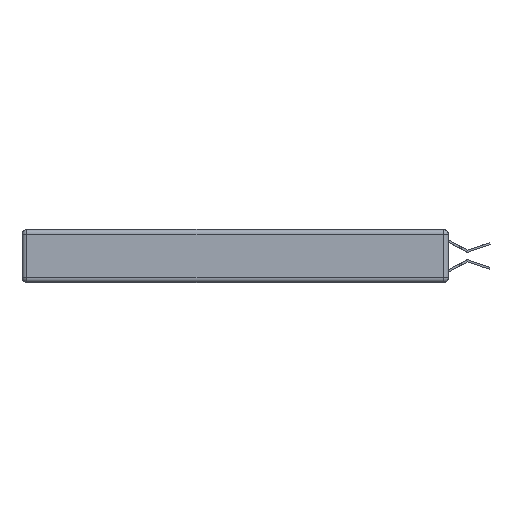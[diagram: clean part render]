
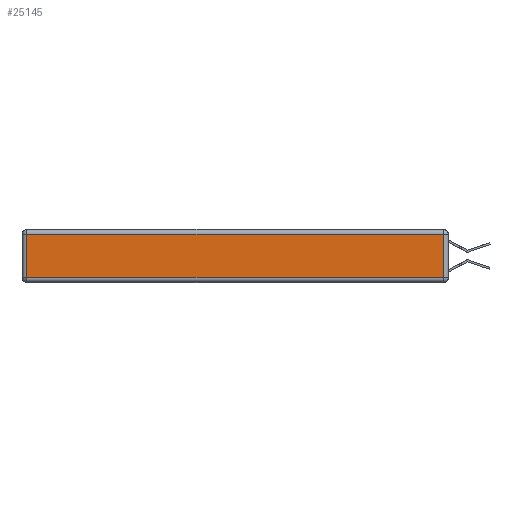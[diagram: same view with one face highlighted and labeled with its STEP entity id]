
A CAD part, left-side view. The second image highlights one B-rep face of the part: STEP entity #25145.
In plain terms, the highlighted planar face has unit normal (-1, 0, 0).
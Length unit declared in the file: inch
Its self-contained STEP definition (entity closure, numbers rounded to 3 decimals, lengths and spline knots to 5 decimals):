
#375 = CARTESIAN_POINT ( 'NONE',  ( 0., 2.75, -0.03 ) ) ;
#379 = ORIENTED_EDGE ( 'NONE', *, *, #14379, .T. ) ;
#1087 = DIRECTION ( 'NONE',  ( 0., 0., 1. ) ) ;
#1217 = DIRECTION ( 'NONE',  ( 0., 0., 1. ) ) ;
#1281 = DIRECTION ( 'NONE',  ( -1., 0., 0. ) ) ;
#1939 = LINE ( 'NONE', #26012, #27994 ) ;
#3780 = LINE ( 'NONE', #12973, #14668 ) ;
#4768 = EDGE_CURVE ( 'NONE', #14205, #11140, #3780, .T. ) ;
#5763 = CARTESIAN_POINT ( 'NONE',  ( 0., 0., -0.343 ) ) ;
#6604 = ORIENTED_EDGE ( 'NONE', *, *, #22451, .T. ) ;
#6844 = DIRECTION ( 'NONE',  ( 0., 1., 0. ) ) ;
#7846 = CARTESIAN_POINT ( 'NONE',  ( 0., 0.03, -0.03 ) ) ;
#10837 = VECTOR ( 'NONE', #6844, 39.37008 ) ;
#10927 = DIRECTION ( 'NONE',  ( 0., -1., 0. ) ) ;
#11140 = VERTEX_POINT ( 'NONE', #18616 ) ;
#12491 = PLANE ( 'NONE',  #12679 ) ;
#12679 = AXIS2_PLACEMENT_3D ( 'NONE', #5763, #1281, #1087 ) ;
#12768 = ORIENTED_EDGE ( 'NONE', *, *, #4768, .T. ) ;
#12973 = CARTESIAN_POINT ( 'NONE',  ( 0., 0., -0.313 ) ) ;
#13622 = ORIENTED_EDGE ( 'NONE', *, *, #28083, .T. ) ;
#13761 = LINE ( 'NONE', #20915, #16245 ) ;
#14205 = VERTEX_POINT ( 'NONE', #19784 ) ;
#14379 = EDGE_CURVE ( 'NONE', #23820, #16287, #23496, .T. ) ;
#14668 = VECTOR ( 'NONE', #10927, 39.37008 ) ;
#16245 = VECTOR ( 'NONE', #25339, 39.37008 ) ;
#16287 = VERTEX_POINT ( 'NONE', #21946 ) ;
#18616 = CARTESIAN_POINT ( 'NONE',  ( 0., 0.03, -0.313 ) ) ;
#19784 = CARTESIAN_POINT ( 'NONE',  ( 0., 2.72, -0.313 ) ) ;
#20915 = CARTESIAN_POINT ( 'NONE',  ( 0., 2.72, -0.343 ) ) ;
#21946 = CARTESIAN_POINT ( 'NONE',  ( 0., 2.72, -0.03 ) ) ;
#22451 = EDGE_CURVE ( 'NONE', #16287, #14205, #13761, .T. ) ;
#22944 = FACE_OUTER_BOUND ( 'NONE', #28021, .T. ) ;
#23496 = LINE ( 'NONE', #375, #10837 ) ;
#23820 = VERTEX_POINT ( 'NONE', #7846 ) ;
#25145 = ADVANCED_FACE ( 'NONE', ( #22944 ), #12491, .T. ) ;
#25339 = DIRECTION ( 'NONE',  ( 0., 0., -1. ) ) ;
#26012 = CARTESIAN_POINT ( 'NONE',  ( 0., 0.03, -0.343 ) ) ;
#27994 = VECTOR ( 'NONE', #1217, 39.37008 ) ;
#28021 = EDGE_LOOP ( 'NONE', ( #12768, #13622, #379, #6604 ) ) ;
#28083 = EDGE_CURVE ( 'NONE', #11140, #23820, #1939, .T. ) ;
